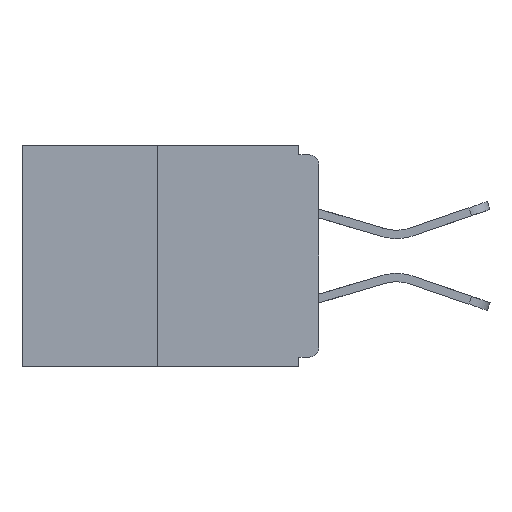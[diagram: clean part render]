
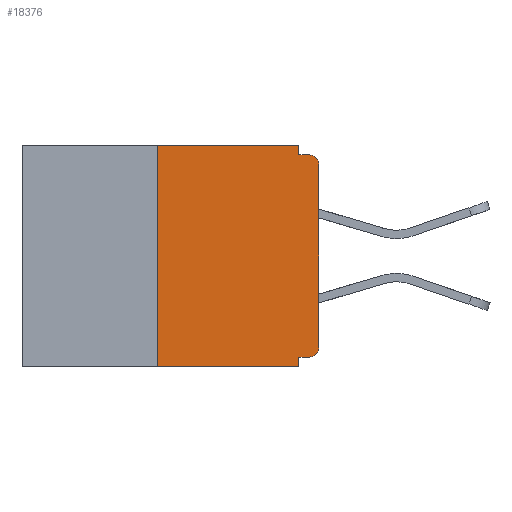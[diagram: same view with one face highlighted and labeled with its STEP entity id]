
A CAD part, left-side view. The second image highlights one B-rep face of the part: STEP entity #18376.
In plain terms, the highlighted planar face has unit normal (-1, 0, 0).
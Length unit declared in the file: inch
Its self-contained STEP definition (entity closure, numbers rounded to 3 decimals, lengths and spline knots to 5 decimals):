
#22 = CARTESIAN_POINT ( 'NONE',  ( 0., 0.031, -0.328 ) ) ;
#219 = LINE ( 'NONE', #18425, #9820 ) ;
#254 = DIRECTION ( 'NONE',  ( -1., 0., 0. ) ) ;
#462 = DIRECTION ( 'NONE',  ( -1., 0., 0. ) ) ;
#494 = DIRECTION ( 'NONE',  ( 0., -1., 0. ) ) ;
#1164 = CARTESIAN_POINT ( 'NONE',  ( 0., 0.015, -0.328 ) ) ;
#1179 = DIRECTION ( 'NONE',  ( 0., 0., 1. ) ) ;
#1427 = ORIENTED_EDGE ( 'NONE', *, *, #3063, .T. ) ;
#1703 = VECTOR ( 'NONE', #6294, 39.37008 ) ;
#1725 = CARTESIAN_POINT ( 'NONE',  ( 0., 0.015, -0.313 ) ) ;
#2030 = VERTEX_POINT ( 'NONE', #3042 ) ;
#2807 = ORIENTED_EDGE ( 'NONE', *, *, #18853, .F. ) ;
#2968 = LINE ( 'NONE', #10425, #3666 ) ;
#3042 = CARTESIAN_POINT ( 'NONE',  ( 0., 0.031, -0.015 ) ) ;
#3063 = EDGE_CURVE ( 'NONE', #4807, #7335, #18640, .T. ) ;
#3253 = CARTESIAN_POINT ( 'NONE',  ( 0., 0., -0.03 ) ) ;
#3469 = EDGE_CURVE ( 'NONE', #11314, #14470, #15565, .T. ) ;
#3666 = VECTOR ( 'NONE', #9978, 39.37008 ) ;
#3770 = ORIENTED_EDGE ( 'NONE', *, *, #9589, .F. ) ;
#4376 = EDGE_CURVE ( 'NONE', #10098, #17004, #11341, .T. ) ;
#4563 = EDGE_CURVE ( 'NONE', #4807, #10098, #7769, .T. ) ;
#4719 = DIRECTION ( 'NONE',  ( 0., 0., -1. ) ) ;
#4792 = CARTESIAN_POINT ( 'NONE',  ( 0., 0.031, 0. ) ) ;
#4807 = VERTEX_POINT ( 'NONE', #18450 ) ;
#4839 = CARTESIAN_POINT ( 'NONE',  ( 0., 0., -0.313 ) ) ;
#5240 = DIRECTION ( 'NONE',  ( 0., -1., 0. ) ) ;
#5873 = VECTOR ( 'NONE', #1179, 39.37008 ) ;
#6294 = DIRECTION ( 'NONE',  ( 0., 0., 1. ) ) ;
#6316 = DIRECTION ( 'NONE',  ( 0., -1., 0. ) ) ;
#6336 = EDGE_CURVE ( 'NONE', #14470, #16970, #10684, .T. ) ;
#6368 = VECTOR ( 'NONE', #6316, 39.37008 ) ;
#6379 = DIRECTION ( 'NONE',  ( 0., 0., -1. ) ) ;
#7335 = VERTEX_POINT ( 'NONE', #9756 ) ;
#7725 = ORIENTED_EDGE ( 'NONE', *, *, #4563, .F. ) ;
#7769 = LINE ( 'NONE', #17858, #5873 ) ;
#7837 = DIRECTION ( 'NONE',  ( 1., 0., 0. ) ) ;
#8257 = ORIENTED_EDGE ( 'NONE', *, *, #16410, .F. ) ;
#9210 = PLANE ( 'NONE',  #18265 ) ;
#9342 = DIRECTION ( 'NONE',  ( 0., 0., -1. ) ) ;
#9458 = CARTESIAN_POINT ( 'NONE',  ( 0., 0., 0. ) ) ;
#9486 = VECTOR ( 'NONE', #16179, 39.37008 ) ;
#9589 = EDGE_CURVE ( 'NONE', #2030, #16970, #14311, .T. ) ;
#9723 = LINE ( 'NONE', #13198, #9486 ) ;
#9756 = CARTESIAN_POINT ( 'NONE',  ( 0., 0.031, -0.343 ) ) ;
#9804 = CARTESIAN_POINT ( 'NONE',  ( 0., 0., -0.015 ) ) ;
#9820 = VECTOR ( 'NONE', #4719, 39.37008 ) ;
#9978 = DIRECTION ( 'NONE',  ( 0., 1., 0. ) ) ;
#10054 = VERTEX_POINT ( 'NONE', #1164 ) ;
#10098 = VERTEX_POINT ( 'NONE', #11491 ) ;
#10325 = VECTOR ( 'NONE', #5240, 39.37008 ) ;
#10425 = CARTESIAN_POINT ( 'NONE',  ( 0., 0., -0.328 ) ) ;
#10528 = ORIENTED_EDGE ( 'NONE', *, *, #18065, .F. ) ;
#10684 = CIRCLE ( 'NONE', #19129, 0.015 ) ;
#10757 = CIRCLE ( 'NONE', #14235, 0.015 ) ;
#11314 = VERTEX_POINT ( 'NONE', #4839 ) ;
#11341 = LINE ( 'NONE', #18472, #12524 ) ;
#11491 = CARTESIAN_POINT ( 'NONE',  ( 0., 0.25, 0. ) ) ;
#11731 = ORIENTED_EDGE ( 'NONE', *, *, #4376, .F. ) ;
#12117 = ORIENTED_EDGE ( 'NONE', *, *, #18367, .T. ) ;
#12127 = CARTESIAN_POINT ( 'NONE',  ( 0., 0.015, -0.015 ) ) ;
#12524 = VECTOR ( 'NONE', #494, 39.37008 ) ;
#13198 = CARTESIAN_POINT ( 'NONE',  ( 0., 0.031, -0.343 ) ) ;
#13841 = CARTESIAN_POINT ( 'NONE',  ( 0., 0.46, 0. ) ) ;
#14102 = FACE_OUTER_BOUND ( 'NONE', #15461, .T. ) ;
#14235 = AXIS2_PLACEMENT_3D ( 'NONE', #1725, #254, #18355 ) ;
#14311 = LINE ( 'NONE', #9804, #10325 ) ;
#14470 = VERTEX_POINT ( 'NONE', #3253 ) ;
#15272 = VERTEX_POINT ( 'NONE', #22 ) ;
#15376 = CARTESIAN_POINT ( 'NONE',  ( 0., 0.015, -0.03 ) ) ;
#15461 = EDGE_LOOP ( 'NONE', ( #11731, #7725, #1427, #10528, #8257, #12117, #17371, #17293, #3770, #2807 ) ) ;
#15565 = LINE ( 'NONE', #9458, #1703 ) ;
#16179 = DIRECTION ( 'NONE',  ( 0., 0., -1. ) ) ;
#16410 = EDGE_CURVE ( 'NONE', #10054, #15272, #2968, .T. ) ;
#16970 = VERTEX_POINT ( 'NONE', #12127 ) ;
#17004 = VERTEX_POINT ( 'NONE', #4792 ) ;
#17293 = ORIENTED_EDGE ( 'NONE', *, *, #6336, .T. ) ;
#17371 = ORIENTED_EDGE ( 'NONE', *, *, #3469, .T. ) ;
#17858 = CARTESIAN_POINT ( 'NONE',  ( 0., 0.25, 0. ) ) ;
#18065 = EDGE_CURVE ( 'NONE', #15272, #7335, #9723, .T. ) ;
#18265 = AXIS2_PLACEMENT_3D ( 'NONE', #13841, #7837, #9342 ) ;
#18355 = DIRECTION ( 'NONE',  ( 0., 0., -1. ) ) ;
#18367 = EDGE_CURVE ( 'NONE', #10054, #11314, #10757, .T. ) ;
#18376 = ADVANCED_FACE ( 'NONE', ( #14102 ), #9210, .F. ) ;
#18425 = CARTESIAN_POINT ( 'NONE',  ( 0., 0.031, 0. ) ) ;
#18436 = CARTESIAN_POINT ( 'NONE',  ( 0., 0.46, -0.343 ) ) ;
#18450 = CARTESIAN_POINT ( 'NONE',  ( 0., 0.25, -0.343 ) ) ;
#18472 = CARTESIAN_POINT ( 'NONE',  ( 0., 0.46, 0. ) ) ;
#18640 = LINE ( 'NONE', #18436, #6368 ) ;
#18853 = EDGE_CURVE ( 'NONE', #17004, #2030, #219, .T. ) ;
#19129 = AXIS2_PLACEMENT_3D ( 'NONE', #15376, #462, #6379 ) ;
